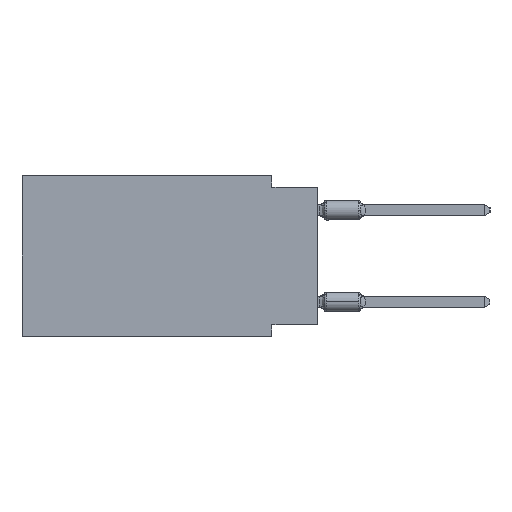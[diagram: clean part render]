
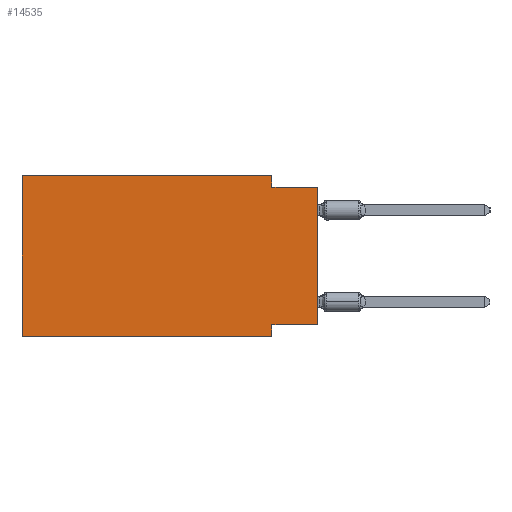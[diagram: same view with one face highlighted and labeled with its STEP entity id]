
A CAD part, left-side view. The second image highlights one B-rep face of the part: STEP entity #14535.
In plain terms, the highlighted planar face has unit normal (-1, 0, 0).
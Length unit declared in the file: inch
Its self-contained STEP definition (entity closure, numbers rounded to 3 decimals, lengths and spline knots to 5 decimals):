
#886 = ORIENTED_EDGE ( 'NONE', *, *, #36157, .F. ) ;
#1113 = VECTOR ( 'NONE', #21563, 39.37008 ) ;
#1598 = VERTEX_POINT ( 'NONE', #40069 ) ;
#2619 = VECTOR ( 'NONE', #52986, 39.37008 ) ;
#4800 = LINE ( 'NONE', #25758, #12264 ) ;
#6733 = VERTEX_POINT ( 'NONE', #40469 ) ;
#6786 = ORIENTED_EDGE ( 'NONE', *, *, #27897, .T. ) ;
#7093 = VECTOR ( 'NONE', #37109, 39.37008 ) ;
#7588 = VECTOR ( 'NONE', #29771, 39.37008 ) ;
#7662 = CARTESIAN_POINT ( 'NONE',  ( 0., 0.645, -0.35 ) ) ;
#7900 = LINE ( 'NONE', #36661, #35373 ) ;
#8119 = LINE ( 'NONE', #8376, #2619 ) ;
#8268 = ORIENTED_EDGE ( 'NONE', *, *, #33462, .F. ) ;
#8376 = CARTESIAN_POINT ( 'NONE',  ( 0., 0., 0. ) ) ;
#8864 = DIRECTION ( 'NONE',  ( 0., 0., -1. ) ) ;
#10142 = AXIS2_PLACEMENT_3D ( 'NONE', #21472, #26326, #8864 ) ;
#10854 = EDGE_CURVE ( 'NONE', #15309, #21338, #35175, .T. ) ;
#11728 = ORIENTED_EDGE ( 'NONE', *, *, #30394, .F. ) ;
#12264 = VECTOR ( 'NONE', #37571, 39.37008 ) ;
#14535 = ADVANCED_FACE ( 'NONE', ( #22271 ), #38406, .F. ) ;
#14669 = CARTESIAN_POINT ( 'NONE',  ( 0., 0.1, -0.35 ) ) ;
#15309 = VERTEX_POINT ( 'NONE', #50672 ) ;
#15992 = CARTESIAN_POINT ( 'NONE',  ( 0., 0., -0.025 ) ) ;
#16231 = DIRECTION ( 'NONE',  ( 0., 0., -1. ) ) ;
#16425 = CARTESIAN_POINT ( 'NONE',  ( 0., 0., -0.325 ) ) ;
#16788 = VERTEX_POINT ( 'NONE', #20900 ) ;
#16909 = EDGE_CURVE ( 'NONE', #18512, #21338, #38602, .T. ) ;
#18512 = VERTEX_POINT ( 'NONE', #7662 ) ;
#20900 = CARTESIAN_POINT ( 'NONE',  ( 0., 0., -0.025 ) ) ;
#21158 = CARTESIAN_POINT ( 'NONE',  ( 0., 0.645, -0.35 ) ) ;
#21338 = VERTEX_POINT ( 'NONE', #14669 ) ;
#21472 = CARTESIAN_POINT ( 'NONE',  ( 0., 0.645, 0. ) ) ;
#21563 = DIRECTION ( 'NONE',  ( 0., 0., -1. ) ) ;
#22271 = FACE_OUTER_BOUND ( 'NONE', #41843, .T. ) ;
#25060 = ORIENTED_EDGE ( 'NONE', *, *, #10854, .F. ) ;
#25758 = CARTESIAN_POINT ( 'NONE',  ( 0., 0.645, 0. ) ) ;
#26326 = DIRECTION ( 'NONE',  ( 1., 0., 0. ) ) ;
#27897 = EDGE_CURVE ( 'NONE', #6733, #16788, #8119, .T. ) ;
#28348 = VERTEX_POINT ( 'NONE', #45108 ) ;
#29771 = DIRECTION ( 'NONE',  ( 0., -1., 0. ) ) ;
#30394 = EDGE_CURVE ( 'NONE', #48215, #1598, #4800, .T. ) ;
#32385 = DIRECTION ( 'NONE',  ( 0., -1., 0. ) ) ;
#32557 = LINE ( 'NONE', #16425, #7093 ) ;
#32640 = VECTOR ( 'NONE', #37743, 39.37008 ) ;
#33462 = EDGE_CURVE ( 'NONE', #18512, #48215, #41779, .T. ) ;
#35175 = LINE ( 'NONE', #41717, #1113 ) ;
#35344 = ORIENTED_EDGE ( 'NONE', *, *, #16909, .T. ) ;
#35373 = VECTOR ( 'NONE', #16231, 39.37008 ) ;
#35771 = EDGE_CURVE ( 'NONE', #1598, #28348, #7900, .T. ) ;
#36157 = EDGE_CURVE ( 'NONE', #6733, #15309, #32557, .T. ) ;
#36661 = CARTESIAN_POINT ( 'NONE',  ( 0., 0.1, 0. ) ) ;
#37109 = DIRECTION ( 'NONE',  ( 0., 1., 0. ) ) ;
#37571 = DIRECTION ( 'NONE',  ( 0., -1., 0. ) ) ;
#37743 = DIRECTION ( 'NONE',  ( 0., 0., 1. ) ) ;
#37750 = VECTOR ( 'NONE', #32385, 39.37008 ) ;
#38406 = PLANE ( 'NONE',  #10142 ) ;
#38548 = CARTESIAN_POINT ( 'NONE',  ( 0., 0.645, 0. ) ) ;
#38602 = LINE ( 'NONE', #21158, #7588 ) ;
#39067 = ORIENTED_EDGE ( 'NONE', *, *, #35771, .F. ) ;
#40069 = CARTESIAN_POINT ( 'NONE',  ( 0., 0.1, 0. ) ) ;
#40469 = CARTESIAN_POINT ( 'NONE',  ( 0., 0., -0.325 ) ) ;
#41717 = CARTESIAN_POINT ( 'NONE',  ( 0., 0.1, -0.35 ) ) ;
#41779 = LINE ( 'NONE', #38548, #32640 ) ;
#41843 = EDGE_LOOP ( 'NONE', ( #6786, #42986, #39067, #11728, #8268, #35344, #25060, #886 ) ) ;
#42986 = ORIENTED_EDGE ( 'NONE', *, *, #49425, .F. ) ;
#45108 = CARTESIAN_POINT ( 'NONE',  ( 0., 0.1, -0.025 ) ) ;
#46790 = CARTESIAN_POINT ( 'NONE',  ( 0., 0.645, 0. ) ) ;
#48215 = VERTEX_POINT ( 'NONE', #46790 ) ;
#49425 = EDGE_CURVE ( 'NONE', #28348, #16788, #52801, .T. ) ;
#50672 = CARTESIAN_POINT ( 'NONE',  ( 0., 0.1, -0.325 ) ) ;
#52801 = LINE ( 'NONE', #15992, #37750 ) ;
#52986 = DIRECTION ( 'NONE',  ( 0., 0., 1. ) ) ;
